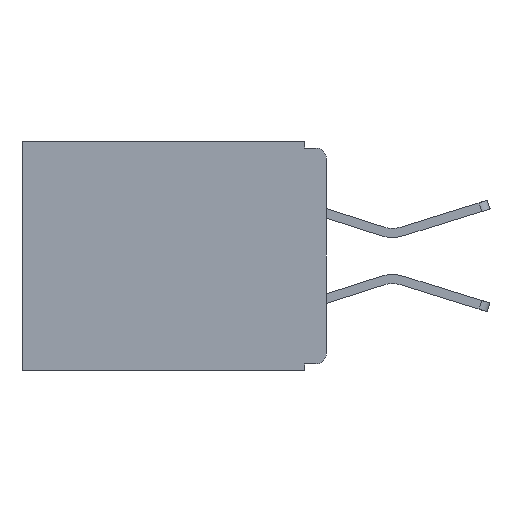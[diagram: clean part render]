
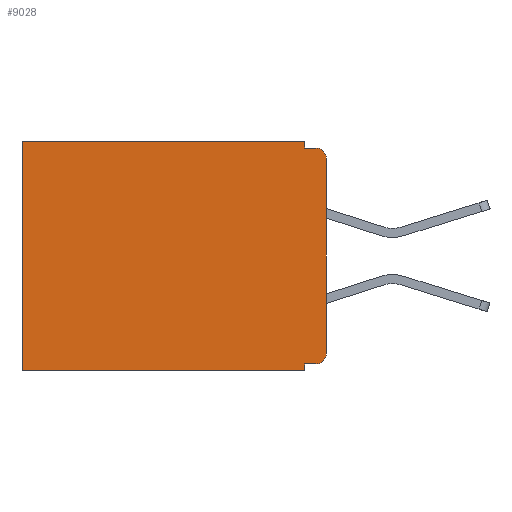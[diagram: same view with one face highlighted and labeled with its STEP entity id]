
A CAD part, left-side view. The second image highlights one B-rep face of the part: STEP entity #9028.
In plain terms, the highlighted planar face has unit normal (-1, 0, 0).
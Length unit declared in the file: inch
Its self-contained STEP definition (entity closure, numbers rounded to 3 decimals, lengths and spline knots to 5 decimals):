
#301 = AXIS2_PLACEMENT_3D ( 'NONE', #17863, #26978, #27004 ) ;
#1039 = CARTESIAN_POINT ( 'NONE',  ( 0.3, 0., -0.32 ) ) ;
#1040 = VERTEX_POINT ( 'NONE', #26172 ) ;
#1238 = CARTESIAN_POINT ( 'NONE',  ( 0.3, 0., -0.305 ) ) ;
#1391 = EDGE_CURVE ( 'NONE', #5019, #18902, #19626, .T. ) ;
#1708 = CARTESIAN_POINT ( 'NONE',  ( 0.3, 0.031, 0. ) ) ;
#1961 = VERTEX_POINT ( 'NONE', #13358 ) ;
#2768 = LINE ( 'NONE', #1708, #25109 ) ;
#2769 = VERTEX_POINT ( 'NONE', #27360 ) ;
#2841 = VERTEX_POINT ( 'NONE', #23147 ) ;
#3158 = CARTESIAN_POINT ( 'NONE',  ( 0.3, 0., -0.33 ) ) ;
#3161 = ORIENTED_EDGE ( 'NONE', *, *, #26072, .F. ) ;
#3315 = DIRECTION ( 'NONE',  ( 0., 1., 0. ) ) ;
#3546 = ORIENTED_EDGE ( 'NONE', *, *, #16010, .F. ) ;
#3746 = ORIENTED_EDGE ( 'NONE', *, *, #1391, .T. ) ;
#3922 = PLANE ( 'NONE',  #8797 ) ;
#4099 = ORIENTED_EDGE ( 'NONE', *, *, #22448, .T. ) ;
#4322 = VERTEX_POINT ( 'NONE', #8211 ) ;
#4328 = FACE_OUTER_BOUND ( 'NONE', #12498, .T. ) ;
#4395 = ORIENTED_EDGE ( 'NONE', *, *, #6229, .F. ) ;
#4762 = EDGE_CURVE ( 'NONE', #1040, #1961, #24182, .T. ) ;
#4819 = EDGE_CURVE ( 'NONE', #4322, #20683, #10092, .T. ) ;
#5011 = CARTESIAN_POINT ( 'NONE',  ( 0.3, 0.015, -0.305 ) ) ;
#5019 = VERTEX_POINT ( 'NONE', #27398 ) ;
#6229 = EDGE_CURVE ( 'NONE', #2841, #11770, #2768, .T. ) ;
#6367 = VECTOR ( 'NONE', #19976, 39.37008 ) ;
#6887 = VECTOR ( 'NONE', #3315, 39.37008 ) ;
#7018 = ORIENTED_EDGE ( 'NONE', *, *, #17777, .F. ) ;
#7146 = ORIENTED_EDGE ( 'NONE', *, *, #4819, .T. ) ;
#7188 = DIRECTION ( 'NONE',  ( 0., 0., -1. ) ) ;
#7351 = EDGE_CURVE ( 'NONE', #2769, #1040, #13294, .T. ) ;
#7412 = CARTESIAN_POINT ( 'NONE',  ( 0.3, 0.437, -0.33 ) ) ;
#7583 = ORIENTED_EDGE ( 'NONE', *, *, #7351, .F. ) ;
#7738 = ORIENTED_EDGE ( 'NONE', *, *, #4762, .F. ) ;
#8211 = CARTESIAN_POINT ( 'NONE',  ( 0.3, 0.437, 0. ) ) ;
#8321 = CARTESIAN_POINT ( 'NONE',  ( 0.3, 0., -0.33 ) ) ;
#8510 = ORIENTED_EDGE ( 'NONE', *, *, #22252, .T. ) ;
#8797 = AXIS2_PLACEMENT_3D ( 'NONE', #8321, #25512, #12670 ) ;
#9028 = ADVANCED_FACE ( 'NONE', ( #4328 ), #3922, .F. ) ;
#9776 = DIRECTION ( 'NONE',  ( 0., 1., 0. ) ) ;
#10092 = LINE ( 'NONE', #7412, #20782 ) ;
#10266 = CARTESIAN_POINT ( 'NONE',  ( 0.3, 0.031, -0.01 ) ) ;
#11060 = VERTEX_POINT ( 'NONE', #1238 ) ;
#11406 = DIRECTION ( 'NONE',  ( 0., -1., 0. ) ) ;
#11770 = VERTEX_POINT ( 'NONE', #10266 ) ;
#12123 = LINE ( 'NONE', #14348, #17163 ) ;
#12159 = AXIS2_PLACEMENT_3D ( 'NONE', #5011, #20040, #7188 ) ;
#12498 = EDGE_LOOP ( 'NONE', ( #3161, #3746, #3546, #4395, #4099, #7146, #7018, #7738, #7583, #8510 ) ) ;
#12670 = DIRECTION ( 'NONE',  ( 0., 0., -1. ) ) ;
#13294 = LINE ( 'NONE', #1039, #6887 ) ;
#13358 = CARTESIAN_POINT ( 'NONE',  ( 0.3, 0.031, -0.33 ) ) ;
#13572 = CARTESIAN_POINT ( 'NONE',  ( 0.3, 0., -0.01 ) ) ;
#14307 = VECTOR ( 'NONE', #9776, 39.37008 ) ;
#14348 = CARTESIAN_POINT ( 'NONE',  ( 0.3, 0., 0. ) ) ;
#15799 = CARTESIAN_POINT ( 'NONE',  ( 0.3, 0.031, -0.33 ) ) ;
#16010 = EDGE_CURVE ( 'NONE', #11770, #18902, #20081, .T. ) ;
#16163 = CIRCLE ( 'NONE', #12159, 0.015 ) ;
#16456 = CARTESIAN_POINT ( 'NONE',  ( 0.3, 0., -0.33 ) ) ;
#16489 = DIRECTION ( 'NONE',  ( 0., 1., 0. ) ) ;
#17163 = VECTOR ( 'NONE', #16489, 39.37008 ) ;
#17777 = EDGE_CURVE ( 'NONE', #1961, #20683, #19970, .T. ) ;
#17863 = CARTESIAN_POINT ( 'NONE',  ( 0.3, 0.015, -0.025 ) ) ;
#18614 = DIRECTION ( 'NONE',  ( 0., 0., -1. ) ) ;
#18902 = VERTEX_POINT ( 'NONE', #26522 ) ;
#18997 = CARTESIAN_POINT ( 'NONE',  ( 0.3, 0.437, -0.33 ) ) ;
#19431 = VECTOR ( 'NONE', #11406, 39.37008 ) ;
#19626 = CIRCLE ( 'NONE', #301, 0.015 ) ;
#19970 = LINE ( 'NONE', #3158, #14307 ) ;
#19976 = DIRECTION ( 'NONE',  ( 0., 0., -1. ) ) ;
#20040 = DIRECTION ( 'NONE',  ( -1., 0., 0. ) ) ;
#20081 = LINE ( 'NONE', #13572, #19431 ) ;
#20683 = VERTEX_POINT ( 'NONE', #18997 ) ;
#20712 = LINE ( 'NONE', #16456, #25784 ) ;
#20782 = VECTOR ( 'NONE', #24599, 39.37008 ) ;
#21185 = DIRECTION ( 'NONE',  ( 0., 0., -1. ) ) ;
#22252 = EDGE_CURVE ( 'NONE', #2769, #11060, #16163, .T. ) ;
#22448 = EDGE_CURVE ( 'NONE', #2841, #4322, #12123, .T. ) ;
#23147 = CARTESIAN_POINT ( 'NONE',  ( 0.3, 0.031, 0. ) ) ;
#24182 = LINE ( 'NONE', #15799, #6367 ) ;
#24599 = DIRECTION ( 'NONE',  ( 0., 0., -1. ) ) ;
#25109 = VECTOR ( 'NONE', #21185, 39.37008 ) ;
#25512 = DIRECTION ( 'NONE',  ( 1., 0., 0. ) ) ;
#25784 = VECTOR ( 'NONE', #18614, 39.37008 ) ;
#26072 = EDGE_CURVE ( 'NONE', #5019, #11060, #20712, .T. ) ;
#26172 = CARTESIAN_POINT ( 'NONE',  ( 0.3, 0.031, -0.32 ) ) ;
#26522 = CARTESIAN_POINT ( 'NONE',  ( 0.3, 0.015, -0.01 ) ) ;
#26978 = DIRECTION ( 'NONE',  ( -1., 0., 0. ) ) ;
#27004 = DIRECTION ( 'NONE',  ( 0., 0., -1. ) ) ;
#27360 = CARTESIAN_POINT ( 'NONE',  ( 0.3, 0.015, -0.32 ) ) ;
#27398 = CARTESIAN_POINT ( 'NONE',  ( 0.3, 0., -0.025 ) ) ;
